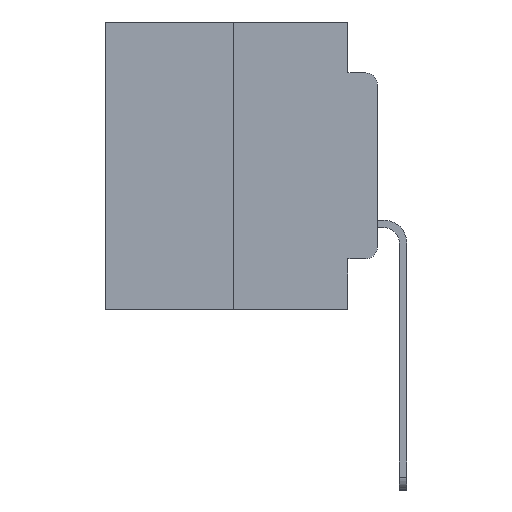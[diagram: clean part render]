
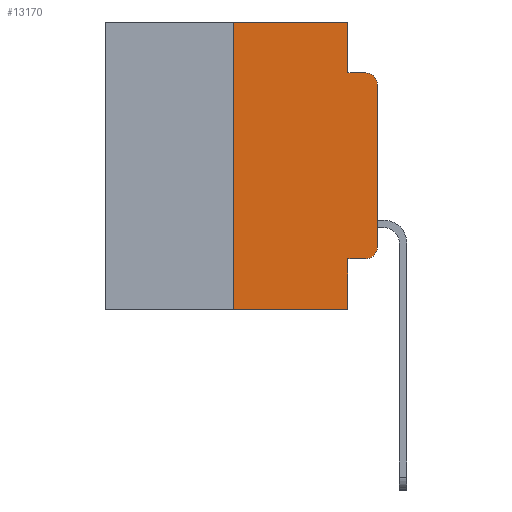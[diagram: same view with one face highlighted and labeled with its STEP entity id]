
A CAD part, left-side view. The second image highlights one B-rep face of the part: STEP entity #13170.
In plain terms, the highlighted planar face has unit normal (-1, 0, 0).
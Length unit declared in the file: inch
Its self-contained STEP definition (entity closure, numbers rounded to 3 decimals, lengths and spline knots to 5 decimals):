
#1165 = ORIENTED_EDGE ( 'NONE', *, *, #2743, .T. ) ;
#1214 = CARTESIAN_POINT ( 'NONE',  ( 0., 0.051, -0.4115 ) ) ;
#1374 = CARTESIAN_POINT ( 'NONE',  ( 0., 0.02, -0.4115 ) ) ;
#1574 = CARTESIAN_POINT ( 'NONE',  ( 0., 0.051, -0.0885 ) ) ;
#1734 = CARTESIAN_POINT ( 'NONE',  ( 0., 0.25, 0. ) ) ;
#1982 = ORIENTED_EDGE ( 'NONE', *, *, #2911, .T. ) ;
#2170 = LINE ( 'NONE', #7960, #23544 ) ;
#2513 = PLANE ( 'NONE',  #16610 ) ;
#2743 = EDGE_CURVE ( 'NONE', #4005, #12348, #23023, .T. ) ;
#2911 = EDGE_CURVE ( 'NONE', #12348, #4940, #8854, .T. ) ;
#3387 = VERTEX_POINT ( 'NONE', #1574 ) ;
#3483 = CARTESIAN_POINT ( 'NONE',  ( 0., 0.051, 0. ) ) ;
#3752 = AXIS2_PLACEMENT_3D ( 'NONE', #20561, #7762, #13985 ) ;
#3953 = CARTESIAN_POINT ( 'NONE',  ( 0., 0.051, 0. ) ) ;
#4005 = VERTEX_POINT ( 'NONE', #12571 ) ;
#4213 = EDGE_CURVE ( 'NONE', #27021, #25714, #14190, .T. ) ;
#4326 = CARTESIAN_POINT ( 'NONE',  ( 0., 0.473, 0. ) ) ;
#4596 = ORIENTED_EDGE ( 'NONE', *, *, #19316, .F. ) ;
#4667 = CARTESIAN_POINT ( 'NONE',  ( 0., 0.02, -0.0885 ) ) ;
#4885 = VECTOR ( 'NONE', #25418, 39.37008 ) ;
#4940 = VERTEX_POINT ( 'NONE', #14563 ) ;
#5796 = CARTESIAN_POINT ( 'NONE',  ( 0., 0.051, -0.0885 ) ) ;
#6090 = DIRECTION ( 'NONE',  ( -1., 0., 0. ) ) ;
#6222 = CARTESIAN_POINT ( 'NONE',  ( 0., 0., 0. ) ) ;
#6348 = AXIS2_PLACEMENT_3D ( 'NONE', #10826, #6090, #15131 ) ;
#6364 = CARTESIAN_POINT ( 'NONE',  ( 0., 0.25, 0. ) ) ;
#6743 = LINE ( 'NONE', #5796, #24353 ) ;
#6768 = VERTEX_POINT ( 'NONE', #24798 ) ;
#7181 = EDGE_CURVE ( 'NONE', #6768, #10199, #14709, .T. ) ;
#7422 = ORIENTED_EDGE ( 'NONE', *, *, #25657, .F. ) ;
#7762 = DIRECTION ( 'NONE',  ( -1., 0., 0. ) ) ;
#7960 = CARTESIAN_POINT ( 'NONE',  ( 0., 0.051, 0. ) ) ;
#8156 = DIRECTION ( 'NONE',  ( 0., 0., -1. ) ) ;
#8854 = CIRCLE ( 'NONE', #6348, 0.02 ) ;
#8867 = ORIENTED_EDGE ( 'NONE', *, *, #11864, .T. ) ;
#8868 = VECTOR ( 'NONE', #25962, 39.37008 ) ;
#9498 = EDGE_CURVE ( 'NONE', #6768, #27021, #22188, .T. ) ;
#9992 = ORIENTED_EDGE ( 'NONE', *, *, #7181, .T. ) ;
#10199 = VERTEX_POINT ( 'NONE', #16979 ) ;
#10493 = LINE ( 'NONE', #6222, #28050 ) ;
#10591 = EDGE_CURVE ( 'NONE', #3387, #23417, #6743, .T. ) ;
#10791 = VECTOR ( 'NONE', #24705, 39.37008 ) ;
#10826 = CARTESIAN_POINT ( 'NONE',  ( 0., 0.02, -0.3915 ) ) ;
#11144 = EDGE_LOOP ( 'NONE', ( #8867, #18988, #18776, #4596, #18048, #21150, #9992, #7422, #1165, #1982 ) ) ;
#11541 = DIRECTION ( 'NONE',  ( 0., 0., 1. ) ) ;
#11864 = EDGE_CURVE ( 'NONE', #4940, #21326, #10493, .T. ) ;
#12348 = VERTEX_POINT ( 'NONE', #1374 ) ;
#12571 = CARTESIAN_POINT ( 'NONE',  ( 0., 0.051, -0.4115 ) ) ;
#12870 = DIRECTION ( 'NONE',  ( 0., 0., 1. ) ) ;
#13000 = EDGE_CURVE ( 'NONE', #21326, #23417, #21811, .T. ) ;
#13170 = ADVANCED_FACE ( 'NONE', ( #14148 ), #2513, .F. ) ;
#13515 = DIRECTION ( 'NONE',  ( 1., 0., 0. ) ) ;
#13632 = VECTOR ( 'NONE', #19216, 39.37008 ) ;
#13985 = DIRECTION ( 'NONE',  ( 0., 0., -1. ) ) ;
#14148 = FACE_OUTER_BOUND ( 'NONE', #11144, .T. ) ;
#14190 = LINE ( 'NONE', #4326, #10791 ) ;
#14563 = CARTESIAN_POINT ( 'NONE',  ( 0., 0., -0.3915 ) ) ;
#14709 = LINE ( 'NONE', #21640, #8868 ) ;
#15131 = DIRECTION ( 'NONE',  ( 0., 0., -1. ) ) ;
#16610 = AXIS2_PLACEMENT_3D ( 'NONE', #22410, #13515, #22506 ) ;
#16979 = CARTESIAN_POINT ( 'NONE',  ( 0., 0.051, -0.5 ) ) ;
#18048 = ORIENTED_EDGE ( 'NONE', *, *, #4213, .F. ) ;
#18776 = ORIENTED_EDGE ( 'NONE', *, *, #10591, .F. ) ;
#18988 = ORIENTED_EDGE ( 'NONE', *, *, #13000, .T. ) ;
#19216 = DIRECTION ( 'NONE',  ( 0., -1., 0. ) ) ;
#19316 = EDGE_CURVE ( 'NONE', #25714, #3387, #26269, .T. ) ;
#19734 = DIRECTION ( 'NONE',  ( 0., -1., 0. ) ) ;
#20561 = CARTESIAN_POINT ( 'NONE',  ( 0., 0.02, -0.1085 ) ) ;
#21150 = ORIENTED_EDGE ( 'NONE', *, *, #9498, .F. ) ;
#21326 = VERTEX_POINT ( 'NONE', #23605 ) ;
#21640 = CARTESIAN_POINT ( 'NONE',  ( 0., 0.473, -0.5 ) ) ;
#21811 = CIRCLE ( 'NONE', #3752, 0.02 ) ;
#22188 = LINE ( 'NONE', #6364, #24276 ) ;
#22410 = CARTESIAN_POINT ( 'NONE',  ( 0., 0.473, 0. ) ) ;
#22506 = DIRECTION ( 'NONE',  ( 0., 0., -1. ) ) ;
#23023 = LINE ( 'NONE', #1214, #13632 ) ;
#23417 = VERTEX_POINT ( 'NONE', #4667 ) ;
#23544 = VECTOR ( 'NONE', #8156, 39.37008 ) ;
#23605 = CARTESIAN_POINT ( 'NONE',  ( 0., 0., -0.1085 ) ) ;
#24276 = VECTOR ( 'NONE', #11541, 39.37008 ) ;
#24353 = VECTOR ( 'NONE', #19734, 39.37008 ) ;
#24705 = DIRECTION ( 'NONE',  ( 0., -1., 0. ) ) ;
#24798 = CARTESIAN_POINT ( 'NONE',  ( 0., 0.25, -0.5 ) ) ;
#25418 = DIRECTION ( 'NONE',  ( 0., 0., -1. ) ) ;
#25657 = EDGE_CURVE ( 'NONE', #4005, #10199, #2170, .T. ) ;
#25714 = VERTEX_POINT ( 'NONE', #3953 ) ;
#25962 = DIRECTION ( 'NONE',  ( 0., -1., 0. ) ) ;
#26269 = LINE ( 'NONE', #3483, #4885 ) ;
#27021 = VERTEX_POINT ( 'NONE', #1734 ) ;
#28050 = VECTOR ( 'NONE', #12870, 39.37008 ) ;
